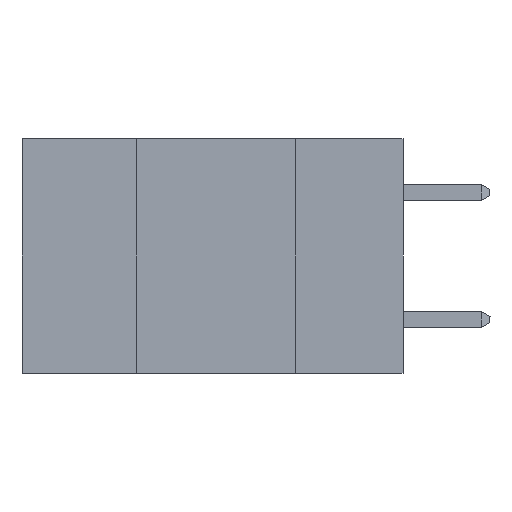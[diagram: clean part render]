
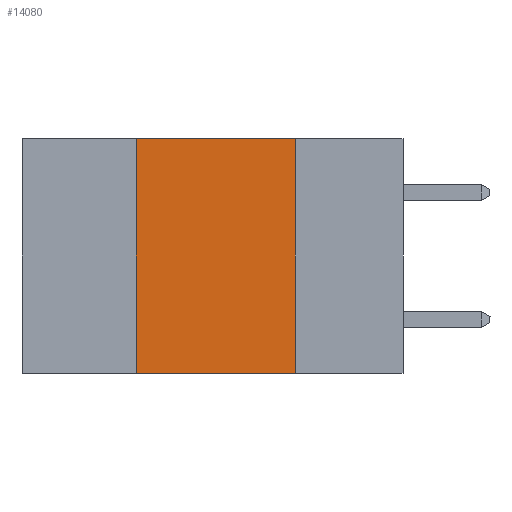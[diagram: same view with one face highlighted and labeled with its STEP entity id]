
A CAD part, left-side view. The second image highlights one B-rep face of the part: STEP entity #14080.
In plain terms, the highlighted planar face has unit normal (-1, 0, 0).
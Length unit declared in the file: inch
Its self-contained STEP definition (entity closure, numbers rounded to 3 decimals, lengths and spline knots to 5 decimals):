
#40 = EDGE_CURVE ( 'NONE', #21313, #39239, #31351, .T. ) ;
#1021 = CARTESIAN_POINT ( 'NONE',  ( 0., 0.6, -0.37 ) ) ;
#1574 = CARTESIAN_POINT ( 'NONE',  ( 0., 0.17, 0. ) ) ;
#1835 = DIRECTION ( 'NONE',  ( 0., 0., 1. ) ) ;
#4387 = EDGE_CURVE ( 'NONE', #21313, #14006, #32370, .T. ) ;
#5106 = VECTOR ( 'NONE', #1835, 39.37008 ) ;
#6835 = LINE ( 'NONE', #1574, #18365 ) ;
#8018 = LINE ( 'NONE', #29396, #11702 ) ;
#8113 = AXIS2_PLACEMENT_3D ( 'NONE', #35197, #14999, #8242 ) ;
#8242 = DIRECTION ( 'NONE',  ( 0., 0., -1. ) ) ;
#9054 = ORIENTED_EDGE ( 'NONE', *, *, #40, .T. ) ;
#9199 = DIRECTION ( 'NONE',  ( 0., -1., 0. ) ) ;
#9655 = CARTESIAN_POINT ( 'NONE',  ( 0., 0.42, -0.37 ) ) ;
#11400 = ORIENTED_EDGE ( 'NONE', *, *, #4387, .F. ) ;
#11702 = VECTOR ( 'NONE', #9199, 39.37008 ) ;
#12115 = CARTESIAN_POINT ( 'NONE',  ( 0., 0.42, 0. ) ) ;
#14006 = VERTEX_POINT ( 'NONE', #34462 ) ;
#14080 = ADVANCED_FACE ( 'NONE', ( #37861 ), #41491, .F. ) ;
#14999 = DIRECTION ( 'NONE',  ( 1., 0., 0. ) ) ;
#16124 = VERTEX_POINT ( 'NONE', #26716 ) ;
#18365 = VECTOR ( 'NONE', #42140, 39.37008 ) ;
#19596 = EDGE_LOOP ( 'NONE', ( #27197, #37366, #11400, #9054 ) ) ;
#20686 = DIRECTION ( 'NONE',  ( 0., -1., 0. ) ) ;
#21313 = VERTEX_POINT ( 'NONE', #9655 ) ;
#23529 = VECTOR ( 'NONE', #20686, 39.37008 ) ;
#26716 = CARTESIAN_POINT ( 'NONE',  ( 0., 0.17, 0. ) ) ;
#27197 = ORIENTED_EDGE ( 'NONE', *, *, #29002, .F. ) ;
#27733 = EDGE_CURVE ( 'NONE', #14006, #16124, #8018, .T. ) ;
#28798 = CARTESIAN_POINT ( 'NONE',  ( 0., 0.17, -0.37 ) ) ;
#29002 = EDGE_CURVE ( 'NONE', #16124, #39239, #6835, .T. ) ;
#29396 = CARTESIAN_POINT ( 'NONE',  ( 0., 0.6, 0. ) ) ;
#31351 = LINE ( 'NONE', #1021, #23529 ) ;
#32370 = LINE ( 'NONE', #12115, #5106 ) ;
#34462 = CARTESIAN_POINT ( 'NONE',  ( 0., 0.42, 0. ) ) ;
#35197 = CARTESIAN_POINT ( 'NONE',  ( 0., 0.6, 0. ) ) ;
#37366 = ORIENTED_EDGE ( 'NONE', *, *, #27733, .F. ) ;
#37861 = FACE_OUTER_BOUND ( 'NONE', #19596, .T. ) ;
#39239 = VERTEX_POINT ( 'NONE', #28798 ) ;
#41491 = PLANE ( 'NONE',  #8113 ) ;
#42140 = DIRECTION ( 'NONE',  ( 0., 0., -1. ) ) ;
